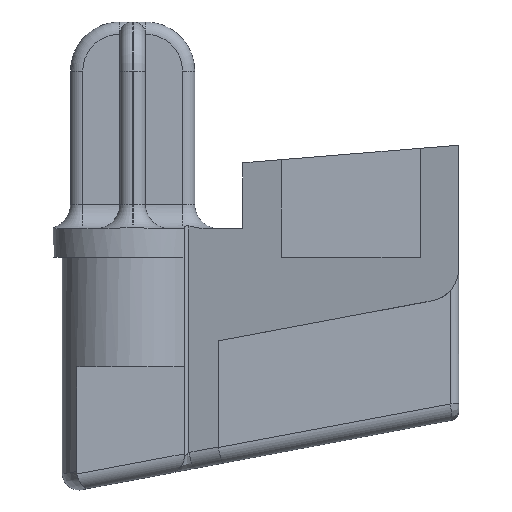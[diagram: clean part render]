
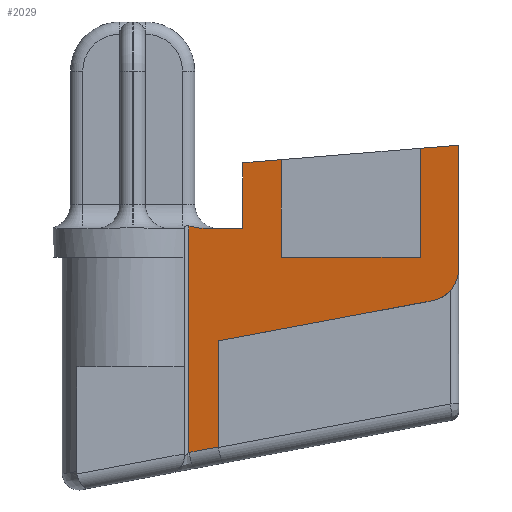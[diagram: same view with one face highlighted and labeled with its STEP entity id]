
A CAD part, left-side view. The second image highlights one B-rep face of the part: STEP entity #2029.
In plain terms, the highlighted planar face has unit normal (-0.982, 0.187, 0).
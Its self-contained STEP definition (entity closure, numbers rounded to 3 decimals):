
#42=PLANE('',#2202);
#214=FACE_OUTER_BOUND('',#337,.T.);
#337=EDGE_LOOP('',(#1506,#1507,#1508,#1509,#1510,#1511,#1512,#1513,#1514,
#1515,#1516,#1517,#1518,#1519,#1520));
#437=B_SPLINE_CURVE_WITH_KNOTS('',3,(#3535,#3536,#3537,#3538,#3539,#3540),
 .UNSPECIFIED.,.F.,.F.,(4,2,4),(-1.566,-1.521,-1.462),
 .UNSPECIFIED.);
#465=ELLIPSE('',#2203,2.036,2.);
#516=LINE('',#3336,#682);
#522=LINE('',#3413,#688);
#524=LINE('',#3426,#690);
#533=LINE('',#3486,#699);
#541=LINE('',#3516,#707);
#542=LINE('',#3519,#708);
#543=LINE('',#3522,#709);
#544=LINE('',#3524,#710);
#545=LINE('',#3526,#711);
#546=LINE('',#3528,#712);
#547=LINE('',#3530,#713);
#548=LINE('',#3532,#714);
#549=LINE('',#3534,#715);
#682=VECTOR('',#2501,10.);
#688=VECTOR('',#2523,10.);
#690=VECTOR('',#2531,10.);
#699=VECTOR('',#2550,10.);
#707=VECTOR('',#2582,10.);
#708=VECTOR('',#2585,10.);
#709=VECTOR('',#2588,10.);
#710=VECTOR('',#2589,10.);
#711=VECTOR('',#2590,10.);
#712=VECTOR('',#2591,10.);
#713=VECTOR('',#2592,10.);
#714=VECTOR('',#2593,10.);
#715=VECTOR('',#2594,10.);
#862=VERTEX_POINT('',#3333);
#863=VERTEX_POINT('',#3335);
#870=VERTEX_POINT('',#3408);
#871=VERTEX_POINT('',#3412);
#873=VERTEX_POINT('',#3425);
#881=VERTEX_POINT('',#3484);
#891=VERTEX_POINT('',#3514);
#892=VERTEX_POINT('',#3518);
#893=VERTEX_POINT('',#3521);
#894=VERTEX_POINT('',#3523);
#895=VERTEX_POINT('',#3525);
#896=VERTEX_POINT('',#3527);
#897=VERTEX_POINT('',#3529);
#898=VERTEX_POINT('',#3531);
#899=VERTEX_POINT('',#3533);
#1074=EDGE_CURVE('',#863,#862,#516,.T.);
#1086=EDGE_CURVE('',#871,#870,#522,.T.);
#1090=EDGE_CURVE('',#870,#873,#524,.T.);
#1104=EDGE_CURVE('',#871,#881,#533,.T.);
#1119=EDGE_CURVE('',#881,#891,#541,.T.);
#1120=EDGE_CURVE('',#891,#892,#542,.T.);
#1121=EDGE_CURVE('',#863,#892,#465,.T.);
#1122=EDGE_CURVE('',#893,#862,#543,.T.);
#1123=EDGE_CURVE('',#894,#893,#544,.T.);
#1124=EDGE_CURVE('',#895,#894,#545,.T.);
#1125=EDGE_CURVE('',#895,#896,#546,.T.);
#1126=EDGE_CURVE('',#897,#896,#547,.T.);
#1127=EDGE_CURVE('',#898,#897,#548,.T.);
#1128=EDGE_CURVE('',#899,#898,#549,.T.);
#1129=EDGE_CURVE('',#899,#873,#437,.F.);
#1506=ORIENTED_EDGE('',*,*,#1120,.T.);
#1507=ORIENTED_EDGE('',*,*,#1121,.F.);
#1508=ORIENTED_EDGE('',*,*,#1074,.T.);
#1509=ORIENTED_EDGE('',*,*,#1122,.F.);
#1510=ORIENTED_EDGE('',*,*,#1123,.F.);
#1511=ORIENTED_EDGE('',*,*,#1124,.F.);
#1512=ORIENTED_EDGE('',*,*,#1125,.T.);
#1513=ORIENTED_EDGE('',*,*,#1126,.F.);
#1514=ORIENTED_EDGE('',*,*,#1127,.F.);
#1515=ORIENTED_EDGE('',*,*,#1128,.F.);
#1516=ORIENTED_EDGE('',*,*,#1129,.T.);
#1517=ORIENTED_EDGE('',*,*,#1090,.F.);
#1518=ORIENTED_EDGE('',*,*,#1086,.F.);
#1519=ORIENTED_EDGE('',*,*,#1104,.T.);
#1520=ORIENTED_EDGE('',*,*,#1119,.T.);
#2029=ADVANCED_FACE('',(#214),#42,.T.);
#2202=AXIS2_PLACEMENT_3D('',#3517,#2583,#2584);
#2203=AXIS2_PLACEMENT_3D('',#3520,#2586,#2587);
#2501=DIRECTION('',(0.,0.,1.));
#2523=DIRECTION('',(0.184,0.966,-0.181));
#2531=DIRECTION('',(0.,0.,1.));
#2550=DIRECTION('',(0.,0.,1.));
#2582=DIRECTION('',(-0.184,-0.966,0.181));
#2583=DIRECTION('center_axis',(-0.982,0.187,0.));
#2584=DIRECTION('ref_axis',(-0.187,-0.982,0.));
#2585=DIRECTION('',(-0.184,-0.966,0.181));
#2586=DIRECTION('center_axis',(0.982,-0.187,0.));
#2587=DIRECTION('ref_axis',(-0.187,-0.982,0.));
#2588=DIRECTION('',(-0.186,-0.979,0.08));
#2589=DIRECTION('',(0.,0.,1.));
#2590=DIRECTION('',(-0.187,-0.982,0.));
#2591=DIRECTION('',(0.,0.,1.));
#2592=DIRECTION('',(-0.186,-0.979,0.08));
#2593=DIRECTION('',(0.,0.,1.));
#2594=DIRECTION('',(-0.187,-0.982,0.));
#3333=CARTESIAN_POINT('',(-10.8,9.8,6.862));
#3335=CARTESIAN_POINT('',(-10.8,9.8,-0.69));
#3336=CARTESIAN_POINT('',(-10.8,9.8,0.));
#3408=CARTESIAN_POINT('',(-7.657,26.303,-11.933));
#3412=CARTESIAN_POINT('',(-8.,24.504,-11.596));
#3413=CARTESIAN_POINT('',(-8.394,22.435,-11.207));
#3425=CARTESIAN_POINT('',(-7.657,26.303,1.919));
#3426=CARTESIAN_POINT('',(-7.657,26.303,0.875));
#3484=CARTESIAN_POINT('',(-8.,24.504,-5.109));
#3486=CARTESIAN_POINT('',(-8.,24.504,-4.945));
#3514=CARTESIAN_POINT('',(-8.75,20.565,-4.37));
#3516=CARTESIAN_POINT('',(-9.645,15.864,-3.488));
#3517=CARTESIAN_POINT('Origin',(-10.352,12.15,0.));
#3518=CARTESIAN_POINT('',(-10.489,11.431,-2.656));
#3519=CARTESIAN_POINT('',(-10.575,10.979,-2.571));
#3520=CARTESIAN_POINT('Origin',(-10.419,11.8,-0.69));
#3521=CARTESIAN_POINT('',(-10.352,12.15,6.671));
#3522=CARTESIAN_POINT('',(-8.193,23.489,5.747));
#3523=CARTESIAN_POINT('',(-10.352,12.15,0.));
#3524=CARTESIAN_POINT('',(-10.352,12.15,3.559));
#3525=CARTESIAN_POINT('',(-8.734,20.65,0.));
#3526=CARTESIAN_POINT('',(-8.661,21.03,0.));
#3527=CARTESIAN_POINT('',(-8.734,20.65,5.978));
#3528=CARTESIAN_POINT('',(-8.734,20.65,0.));
#3529=CARTESIAN_POINT('',(-8.286,23.,5.787));
#3530=CARTESIAN_POINT('',(-7.167,28.88,5.308));
#3531=CARTESIAN_POINT('',(-8.286,23.,1.75));
#3532=CARTESIAN_POINT('',(-8.286,23.,0.));
#3533=CARTESIAN_POINT('',(-7.86,25.238,1.75));
#3534=CARTESIAN_POINT('',(-6.125,34.35,1.75));
#3535=CARTESIAN_POINT('Ctrl Pts',(-7.657,26.303,1.919));
#3536=CARTESIAN_POINT('Ctrl Pts',(-7.687,26.146,1.883));
#3537=CARTESIAN_POINT('Ctrl Pts',(-7.717,25.991,1.845));
#3538=CARTESIAN_POINT('Ctrl Pts',(-7.78,25.658,1.779));
#3539=CARTESIAN_POINT('Ctrl Pts',(-7.824,25.43,1.75));
#3540=CARTESIAN_POINT('Ctrl Pts',(-7.86,25.238,1.75));
